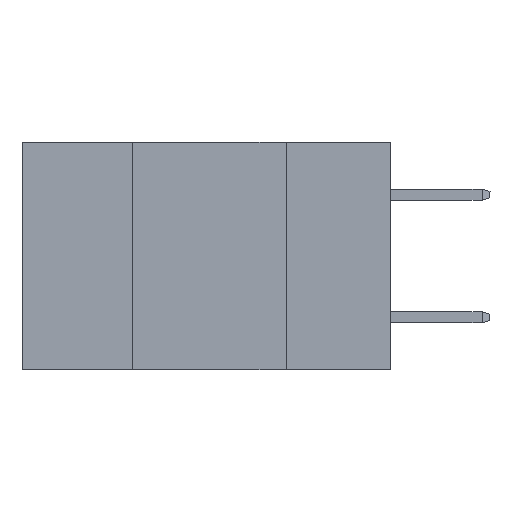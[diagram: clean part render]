
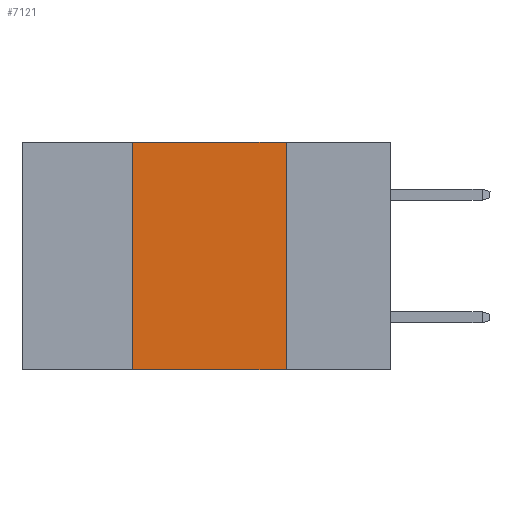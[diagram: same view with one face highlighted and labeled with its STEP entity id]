
A CAD part, left-side view. The second image highlights one B-rep face of the part: STEP entity #7121.
In plain terms, the highlighted planar face has unit normal (-1, 0, 0).
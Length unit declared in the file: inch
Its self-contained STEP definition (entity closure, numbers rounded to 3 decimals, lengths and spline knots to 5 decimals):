
#34 = EDGE_LOOP ( 'NONE', ( #8722, #1882, #4144, #5640 ) ) ;
#121 = CARTESIAN_POINT ( 'NONE',  ( 0., 0.42, 0. ) ) ;
#220 = PLANE ( 'NONE',  #1020 ) ;
#296 = LINE ( 'NONE', #8933, #11380 ) ;
#888 = CARTESIAN_POINT ( 'NONE',  ( 0., 0.6, -0.37 ) ) ;
#1020 = AXIS2_PLACEMENT_3D ( 'NONE', #5637, #2963, #9165 ) ;
#1275 = CARTESIAN_POINT ( 'NONE',  ( 0., 0.6, 0. ) ) ;
#1429 = VECTOR ( 'NONE', #9312, 39.37008 ) ;
#1882 = ORIENTED_EDGE ( 'NONE', *, *, #6067, .F. ) ;
#1900 = VECTOR ( 'NONE', #4527, 39.37008 ) ;
#2725 = DIRECTION ( 'NONE',  ( 0., 0., -1. ) ) ;
#2963 = DIRECTION ( 'NONE',  ( 1., 0., 0. ) ) ;
#3519 = EDGE_CURVE ( 'NONE', #10618, #9523, #4315, .T. ) ;
#3815 = CARTESIAN_POINT ( 'NONE',  ( 0., 0.42, 0. ) ) ;
#4117 = EDGE_CURVE ( 'NONE', #10618, #9401, #9424, .T. ) ;
#4144 = ORIENTED_EDGE ( 'NONE', *, *, #4117, .F. ) ;
#4315 = LINE ( 'NONE', #888, #1900 ) ;
#4527 = DIRECTION ( 'NONE',  ( 0., -1., 0. ) ) ;
#5311 = EDGE_CURVE ( 'NONE', #8134, #9523, #296, .T. ) ;
#5637 = CARTESIAN_POINT ( 'NONE',  ( 0., 0.6, 0. ) ) ;
#5640 = ORIENTED_EDGE ( 'NONE', *, *, #3519, .T. ) ;
#6067 = EDGE_CURVE ( 'NONE', #9401, #8134, #6758, .T. ) ;
#6414 = DIRECTION ( 'NONE',  ( 0., 0., 1. ) ) ;
#6758 = LINE ( 'NONE', #1275, #1429 ) ;
#7121 = ADVANCED_FACE ( 'NONE', ( #11218 ), #220, .F. ) ;
#7334 = VECTOR ( 'NONE', #6414, 39.37008 ) ;
#8134 = VERTEX_POINT ( 'NONE', #10503 ) ;
#8417 = CARTESIAN_POINT ( 'NONE',  ( 0., 0.17, -0.37 ) ) ;
#8722 = ORIENTED_EDGE ( 'NONE', *, *, #5311, .F. ) ;
#8933 = CARTESIAN_POINT ( 'NONE',  ( 0., 0.17, 0. ) ) ;
#9165 = DIRECTION ( 'NONE',  ( 0., 0., -1. ) ) ;
#9312 = DIRECTION ( 'NONE',  ( 0., -1., 0. ) ) ;
#9401 = VERTEX_POINT ( 'NONE', #3815 ) ;
#9424 = LINE ( 'NONE', #121, #7334 ) ;
#9523 = VERTEX_POINT ( 'NONE', #8417 ) ;
#10503 = CARTESIAN_POINT ( 'NONE',  ( 0., 0.17, 0. ) ) ;
#10618 = VERTEX_POINT ( 'NONE', #11604 ) ;
#11218 = FACE_OUTER_BOUND ( 'NONE', #34, .T. ) ;
#11380 = VECTOR ( 'NONE', #2725, 39.37008 ) ;
#11604 = CARTESIAN_POINT ( 'NONE',  ( 0., 0.42, -0.37 ) ) ;
